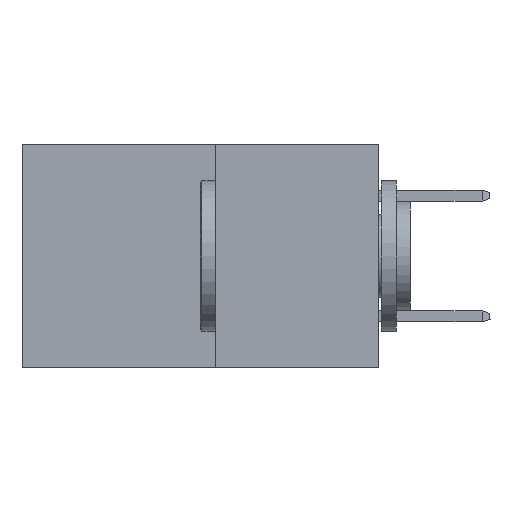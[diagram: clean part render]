
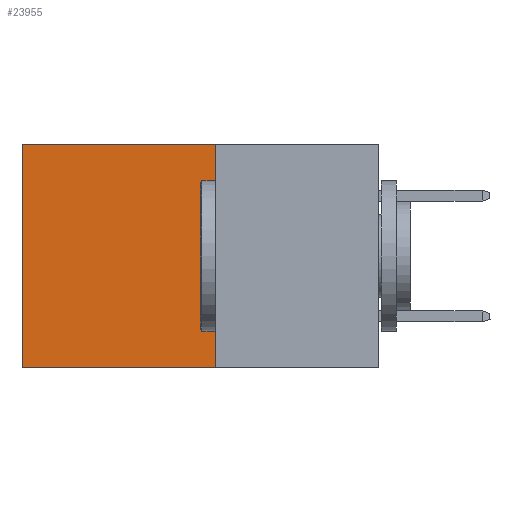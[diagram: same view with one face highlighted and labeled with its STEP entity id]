
A CAD part, left-side view. The second image highlights one B-rep face of the part: STEP entity #23955.
In plain terms, the highlighted planar face has unit normal (-1, 0, 0).
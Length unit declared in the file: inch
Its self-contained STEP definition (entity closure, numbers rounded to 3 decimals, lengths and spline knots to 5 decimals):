
#643 = DIRECTION ( 'NONE',  ( 0., 0., -1. ) ) ;
#936 = VECTOR ( 'NONE', #18971, 39.37008 ) ;
#1543 = EDGE_CURVE ( 'NONE', #28694, #10052, #25918, .T. ) ;
#2951 = CARTESIAN_POINT ( 'NONE',  ( 0.277, 0.59, -0.37 ) ) ;
#4407 = ORIENTED_EDGE ( 'NONE', *, *, #13094, .T. ) ;
#4590 = LINE ( 'NONE', #14939, #29839 ) ;
#5484 = VECTOR ( 'NONE', #22236, 39.37008 ) ;
#7526 = CARTESIAN_POINT ( 'NONE',  ( 0.277, 0.27, -0.37 ) ) ;
#9156 = EDGE_CURVE ( 'NONE', #15012, #9613, #24530, .T. ) ;
#9613 = VERTEX_POINT ( 'NONE', #27665 ) ;
#10052 = VERTEX_POINT ( 'NONE', #2951 ) ;
#10788 = FACE_OUTER_BOUND ( 'NONE', #23385, .T. ) ;
#13094 = EDGE_CURVE ( 'NONE', #9613, #10052, #19242, .T. ) ;
#14722 = DIRECTION ( 'NONE',  ( 0., 0., -1. ) ) ;
#14939 = CARTESIAN_POINT ( 'NONE',  ( 0.277, 0.27, -0.37 ) ) ;
#15012 = VERTEX_POINT ( 'NONE', #27859 ) ;
#17884 = CARTESIAN_POINT ( 'NONE',  ( 0.277, 0.27, -0.37 ) ) ;
#18971 = DIRECTION ( 'NONE',  ( 0., 0., -1. ) ) ;
#19173 = CARTESIAN_POINT ( 'NONE',  ( 0.277, 0.59, -0.37 ) ) ;
#19242 = LINE ( 'NONE', #19173, #936 ) ;
#19454 = PLANE ( 'NONE',  #26677 ) ;
#21765 = ORIENTED_EDGE ( 'NONE', *, *, #1543, .F. ) ;
#21791 = CARTESIAN_POINT ( 'NONE',  ( 0.277, 0.27, 0. ) ) ;
#22236 = DIRECTION ( 'NONE',  ( 0., 1., 0. ) ) ;
#22810 = CARTESIAN_POINT ( 'NONE',  ( 0.277, 0.27, -0.37 ) ) ;
#23385 = EDGE_LOOP ( 'NONE', ( #4407, #21765, #28282, #29177 ) ) ;
#23955 = ADVANCED_FACE ( 'NONE', ( #10788 ), #19454, .F. ) ;
#24530 = LINE ( 'NONE', #21791, #5484 ) ;
#25187 = VECTOR ( 'NONE', #29041, 39.37008 ) ;
#25918 = LINE ( 'NONE', #22810, #25187 ) ;
#26677 = AXIS2_PLACEMENT_3D ( 'NONE', #7526, #28892, #14722 ) ;
#27665 = CARTESIAN_POINT ( 'NONE',  ( 0.277, 0.59, 0. ) ) ;
#27859 = CARTESIAN_POINT ( 'NONE',  ( 0.277, 0.27, 0. ) ) ;
#27998 = EDGE_CURVE ( 'NONE', #15012, #28694, #4590, .T. ) ;
#28282 = ORIENTED_EDGE ( 'NONE', *, *, #27998, .F. ) ;
#28694 = VERTEX_POINT ( 'NONE', #17884 ) ;
#28892 = DIRECTION ( 'NONE',  ( 1., 0., 0. ) ) ;
#29041 = DIRECTION ( 'NONE',  ( 0., 1., 0. ) ) ;
#29177 = ORIENTED_EDGE ( 'NONE', *, *, #9156, .T. ) ;
#29839 = VECTOR ( 'NONE', #643, 39.37008 ) ;
